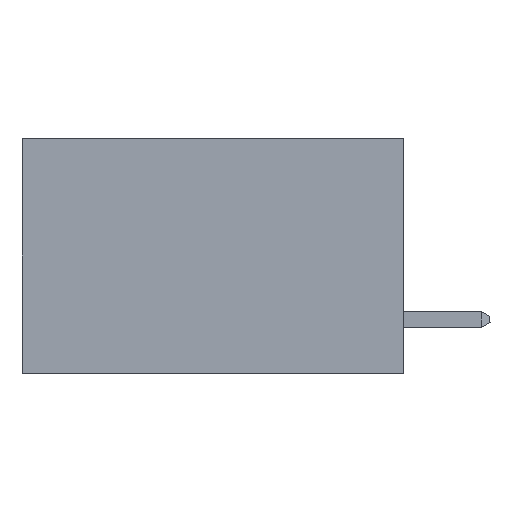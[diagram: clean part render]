
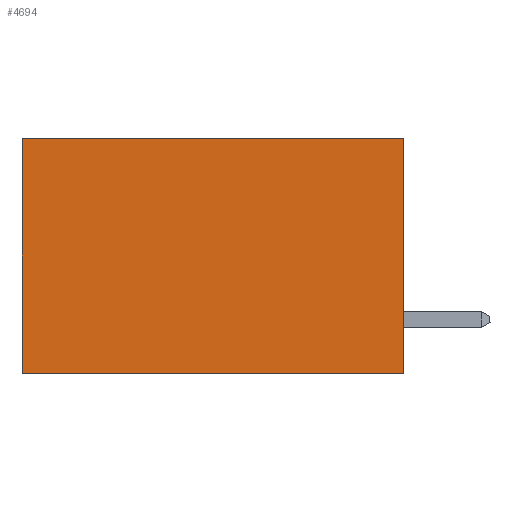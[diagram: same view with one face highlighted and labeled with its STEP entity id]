
A CAD part, left-side view. The second image highlights one B-rep face of the part: STEP entity #4694.
In plain terms, the highlighted planar face has unit normal (-1, 0, 0).
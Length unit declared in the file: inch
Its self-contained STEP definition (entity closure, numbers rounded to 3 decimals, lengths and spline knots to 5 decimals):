
#1144 = DIRECTION ( 'NONE',  ( 0., 0., -1. ) ) ;
#3568 = VERTEX_POINT ( 'NONE', #29917 ) ;
#4694 = ADVANCED_FACE ( 'NONE', ( #6862 ), #22268, .F. ) ;
#4807 = EDGE_CURVE ( 'NONE', #3568, #20792, #34143, .T. ) ;
#6310 = EDGE_CURVE ( 'NONE', #3568, #27686, #38581, .T. ) ;
#6862 = FACE_OUTER_BOUND ( 'NONE', #47998, .T. ) ;
#7540 = DIRECTION ( 'NONE',  ( 1., 0., 0. ) ) ;
#8015 = DIRECTION ( 'NONE',  ( 0., 1., 0. ) ) ;
#10958 = LINE ( 'NONE', #37728, #37060 ) ;
#11721 = CARTESIAN_POINT ( 'NONE',  ( 0.2875, 0., 0. ) ) ;
#14907 = DIRECTION ( 'NONE',  ( 0., 1., 0. ) ) ;
#16133 = VECTOR ( 'NONE', #8015, 39.37008 ) ;
#18806 = EDGE_CURVE ( 'NONE', #20792, #23822, #24116, .T. ) ;
#19334 = CARTESIAN_POINT ( 'NONE',  ( 0.2875, 0., 0. ) ) ;
#20792 = VERTEX_POINT ( 'NONE', #21247 ) ;
#20796 = AXIS2_PLACEMENT_3D ( 'NONE', #47777, #7540, #22116 ) ;
#21085 = EDGE_CURVE ( 'NONE', #27686, #23822, #10958, .T. ) ;
#21247 = CARTESIAN_POINT ( 'NONE',  ( 0.2875, 0.6, 0. ) ) ;
#22116 = DIRECTION ( 'NONE',  ( 0., 0., -1. ) ) ;
#22268 = PLANE ( 'NONE',  #20796 ) ;
#23822 = VERTEX_POINT ( 'NONE', #47886 ) ;
#24116 = LINE ( 'NONE', #33261, #36316 ) ;
#25087 = ORIENTED_EDGE ( 'NONE', *, *, #4807, .T. ) ;
#26115 = DIRECTION ( 'NONE',  ( 0., 0., -1. ) ) ;
#27686 = VERTEX_POINT ( 'NONE', #29881 ) ;
#28738 = VECTOR ( 'NONE', #1144, 39.37008 ) ;
#29881 = CARTESIAN_POINT ( 'NONE',  ( 0.2875, 0., -0.37 ) ) ;
#29917 = CARTESIAN_POINT ( 'NONE',  ( 0.2875, 0., 0. ) ) ;
#33261 = CARTESIAN_POINT ( 'NONE',  ( 0.2875, 0.6, 0. ) ) ;
#34143 = LINE ( 'NONE', #19334, #16133 ) ;
#35529 = ORIENTED_EDGE ( 'NONE', *, *, #18806, .T. ) ;
#36316 = VECTOR ( 'NONE', #26115, 39.37008 ) ;
#37022 = ORIENTED_EDGE ( 'NONE', *, *, #21085, .F. ) ;
#37060 = VECTOR ( 'NONE', #14907, 39.37008 ) ;
#37728 = CARTESIAN_POINT ( 'NONE',  ( 0.2875, 0., -0.37 ) ) ;
#38581 = LINE ( 'NONE', #11721, #28738 ) ;
#46333 = ORIENTED_EDGE ( 'NONE', *, *, #6310, .F. ) ;
#47777 = CARTESIAN_POINT ( 'NONE',  ( 0.2875, 0., 0. ) ) ;
#47886 = CARTESIAN_POINT ( 'NONE',  ( 0.2875, 0.6, -0.37 ) ) ;
#47998 = EDGE_LOOP ( 'NONE', ( #35529, #37022, #46333, #25087 ) ) ;
